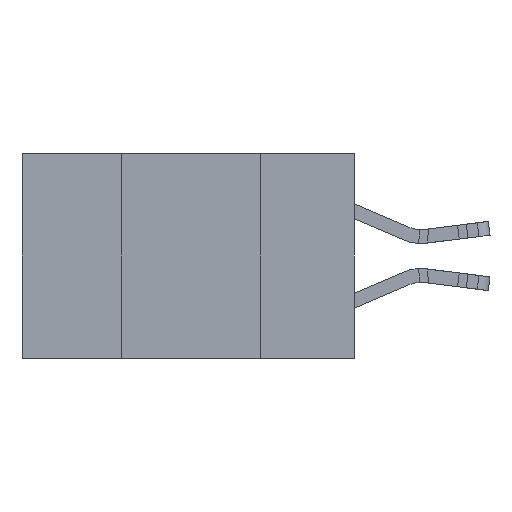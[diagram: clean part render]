
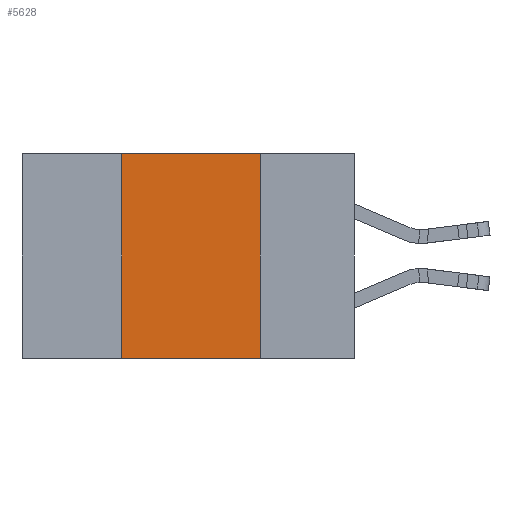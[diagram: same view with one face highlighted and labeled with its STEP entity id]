
A CAD part, left-side view. The second image highlights one B-rep face of the part: STEP entity #5628.
In plain terms, the highlighted planar face has unit normal (-1, 0, 0).
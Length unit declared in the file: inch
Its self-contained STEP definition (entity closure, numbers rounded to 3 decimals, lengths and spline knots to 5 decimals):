
#705 = EDGE_CURVE ( 'NONE', #1166, #11656, #21815, .T. ) ;
#817 = ORIENTED_EDGE ( 'NONE', *, *, #5082, .F. ) ;
#887 = LINE ( 'NONE', #14157, #6331 ) ;
#899 = FACE_OUTER_BOUND ( 'NONE', #3759, .T. ) ;
#1110 = LINE ( 'NONE', #25203, #18665 ) ;
#1166 = VERTEX_POINT ( 'NONE', #18307 ) ;
#1342 = DIRECTION ( 'NONE',  ( 0., -1., 0. ) ) ;
#1880 = DIRECTION ( 'NONE',  ( 0., 0., -1. ) ) ;
#3559 = CARTESIAN_POINT ( 'NONE',  ( 0., 0.42, 0. ) ) ;
#3759 = EDGE_LOOP ( 'NONE', ( #14180, #817, #28655, #19576 ) ) ;
#5082 = EDGE_CURVE ( 'NONE', #6481, #1166, #27068, .T. ) ;
#5628 = ADVANCED_FACE ( 'NONE', ( #899 ), #21210, .F. ) ;
#6331 = VECTOR ( 'NONE', #18614, 39.37008 ) ;
#6481 = VERTEX_POINT ( 'NONE', #3559 ) ;
#6806 = CARTESIAN_POINT ( 'NONE',  ( 0., 0.6, 0. ) ) ;
#6914 = EDGE_CURVE ( 'NONE', #13409, #6481, #1110, .T. ) ;
#7730 = DIRECTION ( 'NONE',  ( 1., 0., 0. ) ) ;
#9326 = VECTOR ( 'NONE', #1342, 39.37008 ) ;
#10673 = VECTOR ( 'NONE', #1880, 39.37008 ) ;
#11533 = CARTESIAN_POINT ( 'NONE',  ( 0., 0.17, 0. ) ) ;
#11656 = VERTEX_POINT ( 'NONE', #15016 ) ;
#11919 = DIRECTION ( 'NONE',  ( 0., 0., 1. ) ) ;
#13409 = VERTEX_POINT ( 'NONE', #20980 ) ;
#14157 = CARTESIAN_POINT ( 'NONE',  ( 0., 0.6, -0.37 ) ) ;
#14180 = ORIENTED_EDGE ( 'NONE', *, *, #705, .F. ) ;
#15016 = CARTESIAN_POINT ( 'NONE',  ( 0., 0.17, -0.37 ) ) ;
#18307 = CARTESIAN_POINT ( 'NONE',  ( 0., 0.17, 0. ) ) ;
#18614 = DIRECTION ( 'NONE',  ( 0., -1., 0. ) ) ;
#18665 = VECTOR ( 'NONE', #11919, 39.37008 ) ;
#19232 = AXIS2_PLACEMENT_3D ( 'NONE', #27742, #7730, #23421 ) ;
#19576 = ORIENTED_EDGE ( 'NONE', *, *, #24996, .T. ) ;
#20980 = CARTESIAN_POINT ( 'NONE',  ( 0., 0.42, -0.37 ) ) ;
#21210 = PLANE ( 'NONE',  #19232 ) ;
#21815 = LINE ( 'NONE', #11533, #10673 ) ;
#23421 = DIRECTION ( 'NONE',  ( 0., 0., -1. ) ) ;
#24996 = EDGE_CURVE ( 'NONE', #13409, #11656, #887, .T. ) ;
#25203 = CARTESIAN_POINT ( 'NONE',  ( 0., 0.42, 0. ) ) ;
#27068 = LINE ( 'NONE', #6806, #9326 ) ;
#27742 = CARTESIAN_POINT ( 'NONE',  ( 0., 0.6, 0. ) ) ;
#28655 = ORIENTED_EDGE ( 'NONE', *, *, #6914, .F. ) ;
